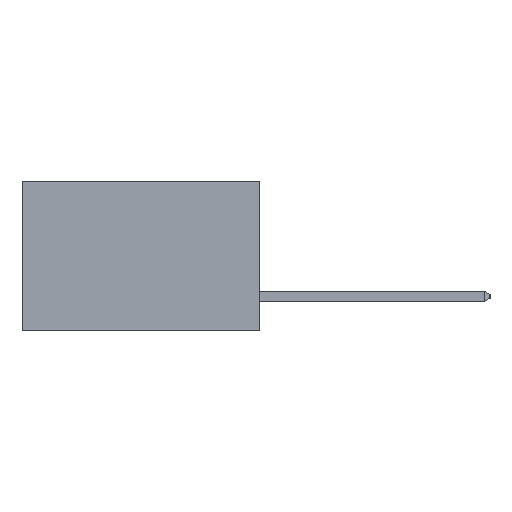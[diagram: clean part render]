
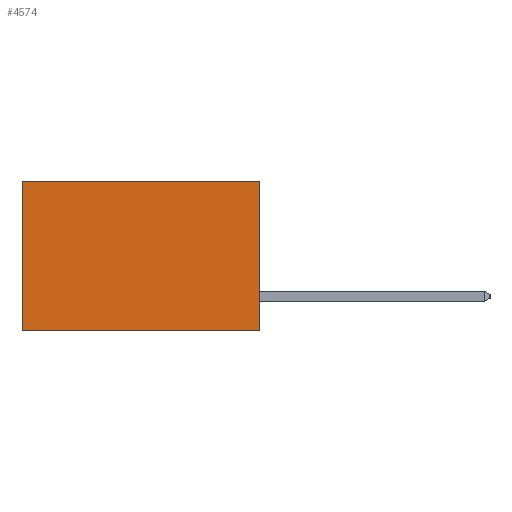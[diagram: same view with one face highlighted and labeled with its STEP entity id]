
A CAD part, left-side view. The second image highlights one B-rep face of the part: STEP entity #4574.
In plain terms, the highlighted planar face has unit normal (-1, 0, 0).
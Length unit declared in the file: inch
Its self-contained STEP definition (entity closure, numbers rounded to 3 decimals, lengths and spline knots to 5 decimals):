
#756 = AXIS2_PLACEMENT_3D ( 'NONE', #1493, #1585, #1546 ) ;
#1265 = DIRECTION ( 'NONE',  ( 0., 0., -1. ) ) ;
#1395 = CARTESIAN_POINT ( 'NONE',  ( 0.277, 0., -0.37 ) ) ;
#1493 = CARTESIAN_POINT ( 'NONE',  ( 0.277, 0., -0.37 ) ) ;
#1502 = CARTESIAN_POINT ( 'NONE',  ( 0.277, 0., 0. ) ) ;
#1546 = DIRECTION ( 'NONE',  ( 0., 0., -1. ) ) ;
#1585 = DIRECTION ( 'NONE',  ( 1., 0., 0. ) ) ;
#1666 = EDGE_CURVE ( 'NONE', #7996, #6562, #7046, .T. ) ;
#2096 = CARTESIAN_POINT ( 'NONE',  ( 0.277, 0., -0.37 ) ) ;
#2304 = DIRECTION ( 'NONE',  ( 0., 1., 0. ) ) ;
#3194 = EDGE_LOOP ( 'NONE', ( #6142, #15125, #12663, #3709 ) ) ;
#3709 = ORIENTED_EDGE ( 'NONE', *, *, #14332, .T. ) ;
#4461 = VERTEX_POINT ( 'NONE', #6280 ) ;
#4574 = ADVANCED_FACE ( 'NONE', ( #14991 ), #6120, .F. ) ;
#5177 = CARTESIAN_POINT ( 'NONE',  ( 0.277, 0.59, -0.37 ) ) ;
#5731 = LINE ( 'NONE', #1395, #7416 ) ;
#5909 = EDGE_CURVE ( 'NONE', #4461, #6562, #8541, .T. ) ;
#5952 = EDGE_CURVE ( 'NONE', #13720, #4461, #5731, .T. ) ;
#6120 = PLANE ( 'NONE',  #756 ) ;
#6142 = ORIENTED_EDGE ( 'NONE', *, *, #1666, .T. ) ;
#6280 = CARTESIAN_POINT ( 'NONE',  ( 0.277, 0., -0.37 ) ) ;
#6562 = VERTEX_POINT ( 'NONE', #9908 ) ;
#6605 = CARTESIAN_POINT ( 'NONE',  ( 0.277, 0., 0. ) ) ;
#7046 = LINE ( 'NONE', #5177, #12798 ) ;
#7416 = VECTOR ( 'NONE', #1265, 39.37008 ) ;
#7996 = VERTEX_POINT ( 'NONE', #11510 ) ;
#8541 = LINE ( 'NONE', #2096, #14441 ) ;
#8805 = DIRECTION ( 'NONE',  ( 0., 1., 0. ) ) ;
#9908 = CARTESIAN_POINT ( 'NONE',  ( 0.277, 0.59, -0.37 ) ) ;
#10752 = DIRECTION ( 'NONE',  ( 0., 0., -1. ) ) ;
#10815 = VECTOR ( 'NONE', #8805, 39.37008 ) ;
#11510 = CARTESIAN_POINT ( 'NONE',  ( 0.277, 0.59, 0. ) ) ;
#12663 = ORIENTED_EDGE ( 'NONE', *, *, #5952, .F. ) ;
#12798 = VECTOR ( 'NONE', #10752, 39.37008 ) ;
#13700 = LINE ( 'NONE', #1502, #10815 ) ;
#13720 = VERTEX_POINT ( 'NONE', #6605 ) ;
#14332 = EDGE_CURVE ( 'NONE', #13720, #7996, #13700, .T. ) ;
#14441 = VECTOR ( 'NONE', #2304, 39.37008 ) ;
#14991 = FACE_OUTER_BOUND ( 'NONE', #3194, .T. ) ;
#15125 = ORIENTED_EDGE ( 'NONE', *, *, #5909, .F. ) ;
